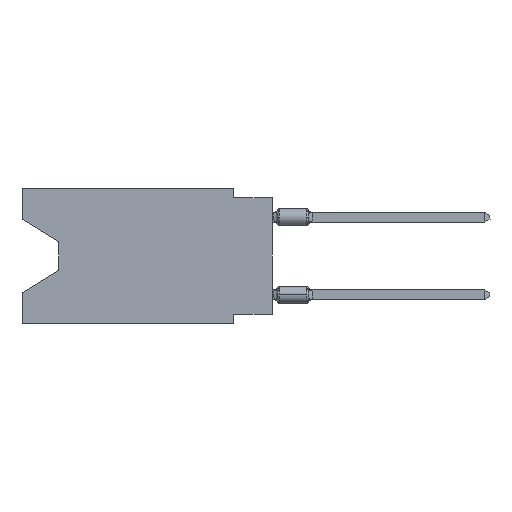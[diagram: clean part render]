
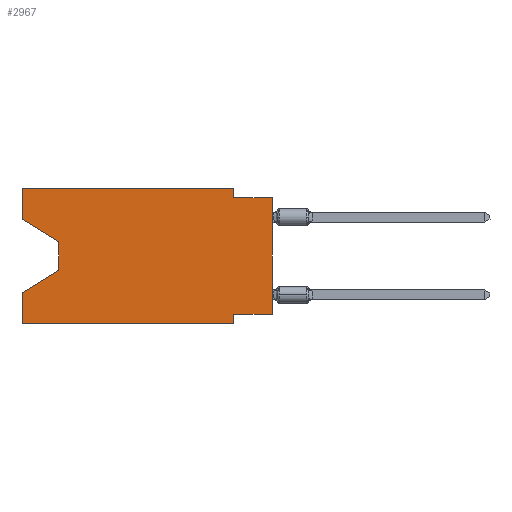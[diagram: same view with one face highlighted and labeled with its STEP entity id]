
A CAD part, left-side view. The second image highlights one B-rep face of the part: STEP entity #2967.
In plain terms, the highlighted planar face has unit normal (-1, 0, 0).
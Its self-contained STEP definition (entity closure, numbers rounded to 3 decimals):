
#372 = CARTESIAN_POINT ( 'NONE',  ( 0., 2.54, 0. ) ) ;
#418 = LINE ( 'NONE', #7315, #10087 ) ;
#945 = EDGE_CURVE ( 'NONE', #3064, #4063, #9072, .T. ) ;
#1151 = DIRECTION ( 'NONE',  ( 0., 0., 1. ) ) ;
#1207 = CARTESIAN_POINT ( 'NONE',  ( 0., 16.383, -8.89 ) ) ;
#1298 = VECTOR ( 'NONE', #1151, 1000. ) ;
#1504 = CARTESIAN_POINT ( 'NONE',  ( 0., 16.383, 0. ) ) ;
#1510 = CARTESIAN_POINT ( 'NONE',  ( 0., 2.54, -8.89 ) ) ;
#1592 = VERTEX_POINT ( 'NONE', #15326 ) ;
#1666 = AXIS2_PLACEMENT_3D ( 'NONE', #2888, #16394, #11309 ) ;
#1724 = CARTESIAN_POINT ( 'NONE',  ( 0., 2.54, 0. ) ) ;
#1767 = LINE ( 'NONE', #372, #7601 ) ;
#1991 = EDGE_CURVE ( 'NONE', #13177, #8521, #17720, .T. ) ;
#2012 = VECTOR ( 'NONE', #11885, 1000. ) ;
#2568 = EDGE_CURVE ( 'NONE', #14006, #13822, #13751, .T. ) ;
#2655 = CARTESIAN_POINT ( 'NONE',  ( 0., 13.97, -3.505 ) ) ;
#2722 = ORIENTED_EDGE ( 'NONE', *, *, #7913, .T. ) ;
#2888 = CARTESIAN_POINT ( 'NONE',  ( 0., 16.383, 0. ) ) ;
#2967 = ADVANCED_FACE ( 'NONE', ( #10030 ), #17005, .F. ) ;
#3064 = VERTEX_POINT ( 'NONE', #7726 ) ;
#3110 = CARTESIAN_POINT ( 'NONE',  ( 0., 0., -0.635 ) ) ;
#3279 = ORIENTED_EDGE ( 'NONE', *, *, #17367, .F. ) ;
#3340 = CARTESIAN_POINT ( 'NONE',  ( 0., 2.54, -8.255 ) ) ;
#3438 = CARTESIAN_POINT ( 'NONE',  ( 0., 16.383, -2.038 ) ) ;
#3914 = LINE ( 'NONE', #18042, #16942 ) ;
#4019 = VECTOR ( 'NONE', #18162, 1000. ) ;
#4044 = CARTESIAN_POINT ( 'NONE',  ( 0., 2.54, -8.89 ) ) ;
#4063 = VERTEX_POINT ( 'NONE', #7684 ) ;
#4138 = EDGE_CURVE ( 'NONE', #13822, #15905, #3914, .T. ) ;
#4264 = VERTEX_POINT ( 'NONE', #12802 ) ;
#4346 = CARTESIAN_POINT ( 'NONE',  ( 0., 16.383, -6.852 ) ) ;
#4359 = ORIENTED_EDGE ( 'NONE', *, *, #2568, .T. ) ;
#5074 = ORIENTED_EDGE ( 'NONE', *, *, #13841, .F. ) ;
#5107 = EDGE_CURVE ( 'NONE', #12136, #4264, #1767, .T. ) ;
#5629 = LINE ( 'NONE', #11307, #17684 ) ;
#5854 = ORIENTED_EDGE ( 'NONE', *, *, #1991, .F. ) ;
#6046 = LINE ( 'NONE', #3110, #9934 ) ;
#6229 = ORIENTED_EDGE ( 'NONE', *, *, #12278, .F. ) ;
#6432 = ORIENTED_EDGE ( 'NONE', *, *, #4138, .T. ) ;
#6794 = DIRECTION ( 'NONE',  ( 0., -1., 0. ) ) ;
#6843 = DIRECTION ( 'NONE',  ( 0., 0.855, -0.519 ) ) ;
#7043 = DIRECTION ( 'NONE',  ( 0., 0., 1. ) ) ;
#7315 = CARTESIAN_POINT ( 'NONE',  ( 0., 16.383, 0. ) ) ;
#7440 = DIRECTION ( 'NONE',  ( 0., 0., -1. ) ) ;
#7601 = VECTOR ( 'NONE', #7440, 1000. ) ;
#7684 = CARTESIAN_POINT ( 'NONE',  ( 0., 0., -0.635 ) ) ;
#7726 = CARTESIAN_POINT ( 'NONE',  ( 0., 0., -8.255 ) ) ;
#7913 = EDGE_CURVE ( 'NONE', #17242, #8521, #13773, .T. ) ;
#8390 = LINE ( 'NONE', #1504, #1298 ) ;
#8399 = EDGE_LOOP ( 'NONE', ( #11098, #4359, #6432, #5074, #2722, #5854, #3279, #13107, #15740, #10543, #9527, #6229 ) ) ;
#8521 = VERTEX_POINT ( 'NONE', #1510 ) ;
#9072 = LINE ( 'NONE', #9156, #2012 ) ;
#9156 = CARTESIAN_POINT ( 'NONE',  ( 0., 0., 0. ) ) ;
#9527 = ORIENTED_EDGE ( 'NONE', *, *, #12162, .F. ) ;
#9717 = LINE ( 'NONE', #12820, #15082 ) ;
#9934 = VECTOR ( 'NONE', #17239, 1000. ) ;
#10030 = FACE_OUTER_BOUND ( 'NONE', #8399, .T. ) ;
#10071 = CARTESIAN_POINT ( 'NONE',  ( 0., 13.97, -3.505 ) ) ;
#10087 = VECTOR ( 'NONE', #11614, 1000. ) ;
#10457 = EDGE_CURVE ( 'NONE', #4264, #4063, #6046, .T. ) ;
#10543 = ORIENTED_EDGE ( 'NONE', *, *, #5107, .F. ) ;
#11098 = ORIENTED_EDGE ( 'NONE', *, *, #14110, .T. ) ;
#11298 = VECTOR ( 'NONE', #12154, 1000. ) ;
#11307 = CARTESIAN_POINT ( 'NONE',  ( 0., 0., -8.255 ) ) ;
#11309 = DIRECTION ( 'NONE',  ( 0., 0., -1. ) ) ;
#11614 = DIRECTION ( 'NONE',  ( 0., -1., 0. ) ) ;
#11885 = DIRECTION ( 'NONE',  ( 0., 0., 1. ) ) ;
#12071 = LINE ( 'NONE', #13620, #11298 ) ;
#12136 = VERTEX_POINT ( 'NONE', #1724 ) ;
#12154 = DIRECTION ( 'NONE',  ( 0., -0.855, -0.519 ) ) ;
#12162 = EDGE_CURVE ( 'NONE', #1592, #12136, #418, .T. ) ;
#12278 = EDGE_CURVE ( 'NONE', #13324, #1592, #8390, .T. ) ;
#12802 = CARTESIAN_POINT ( 'NONE',  ( 0., 2.54, -0.635 ) ) ;
#12820 = CARTESIAN_POINT ( 'NONE',  ( 0., 16.383, 0. ) ) ;
#13107 = ORIENTED_EDGE ( 'NONE', *, *, #945, .T. ) ;
#13177 = VERTEX_POINT ( 'NONE', #3340 ) ;
#13324 = VERTEX_POINT ( 'NONE', #3438 ) ;
#13620 = CARTESIAN_POINT ( 'NONE',  ( 0., 16.383, -2.038 ) ) ;
#13703 = CARTESIAN_POINT ( 'NONE',  ( 0., 16.383, -8.89 ) ) ;
#13751 = LINE ( 'NONE', #2655, #16003 ) ;
#13773 = LINE ( 'NONE', #1207, #16319 ) ;
#13822 = VERTEX_POINT ( 'NONE', #16580 ) ;
#13841 = EDGE_CURVE ( 'NONE', #17242, #15905, #9717, .T. ) ;
#14006 = VERTEX_POINT ( 'NONE', #10071 ) ;
#14110 = EDGE_CURVE ( 'NONE', #13324, #14006, #12071, .T. ) ;
#14139 = DIRECTION ( 'NONE',  ( 0., 1., 0. ) ) ;
#15082 = VECTOR ( 'NONE', #7043, 1000. ) ;
#15326 = CARTESIAN_POINT ( 'NONE',  ( 0., 16.383, 0. ) ) ;
#15740 = ORIENTED_EDGE ( 'NONE', *, *, #10457, .F. ) ;
#15905 = VERTEX_POINT ( 'NONE', #4346 ) ;
#16003 = VECTOR ( 'NONE', #16683, 1000. ) ;
#16319 = VECTOR ( 'NONE', #6794, 1000. ) ;
#16394 = DIRECTION ( 'NONE',  ( 1., 0., 0. ) ) ;
#16580 = CARTESIAN_POINT ( 'NONE',  ( 0., 13.97, -5.385 ) ) ;
#16683 = DIRECTION ( 'NONE',  ( 0., 0., -1. ) ) ;
#16942 = VECTOR ( 'NONE', #6843, 1000. ) ;
#17005 = PLANE ( 'NONE',  #1666 ) ;
#17239 = DIRECTION ( 'NONE',  ( 0., -1., 0. ) ) ;
#17242 = VERTEX_POINT ( 'NONE', #13703 ) ;
#17367 = EDGE_CURVE ( 'NONE', #3064, #13177, #5629, .T. ) ;
#17684 = VECTOR ( 'NONE', #14139, 1000. ) ;
#17720 = LINE ( 'NONE', #4044, #4019 ) ;
#18042 = CARTESIAN_POINT ( 'NONE',  ( 0., 13.97, -5.385 ) ) ;
#18162 = DIRECTION ( 'NONE',  ( 0., 0., -1. ) ) ;
